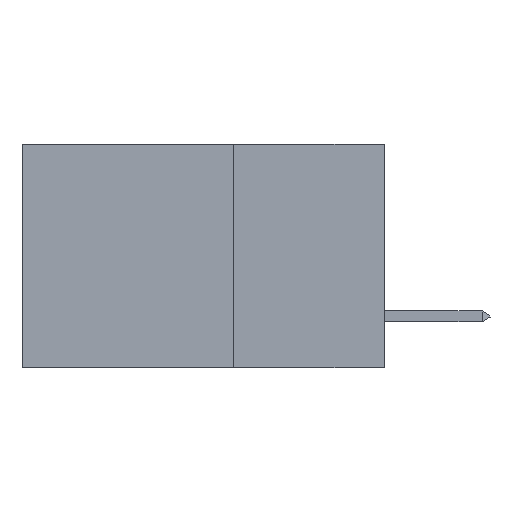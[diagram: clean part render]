
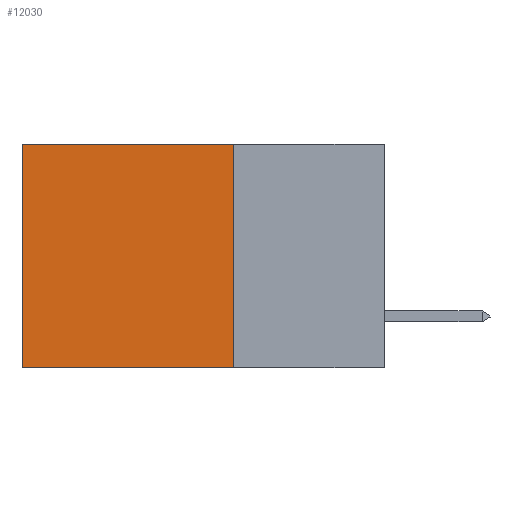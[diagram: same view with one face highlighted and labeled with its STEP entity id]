
A CAD part, left-side view. The second image highlights one B-rep face of the part: STEP entity #12030.
In plain terms, the highlighted planar face has unit normal (-1, 0, 0).
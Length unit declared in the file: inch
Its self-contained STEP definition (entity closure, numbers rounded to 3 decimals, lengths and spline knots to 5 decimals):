
#408 = CARTESIAN_POINT ( 'NONE',  ( 0.2875, 0.25, 0. ) ) ;
#1227 = FACE_OUTER_BOUND ( 'NONE', #35162, .T. ) ;
#2626 = LINE ( 'NONE', #7851, #26448 ) ;
#3284 = VERTEX_POINT ( 'NONE', #4721 ) ;
#3836 = DIRECTION ( 'NONE',  ( 0., 1., 0. ) ) ;
#4527 = PLANE ( 'NONE',  #27388 ) ;
#4721 = CARTESIAN_POINT ( 'NONE',  ( 0.2875, 0.25, -0.37 ) ) ;
#6178 = VECTOR ( 'NONE', #39153, 39.37008 ) ;
#7851 = CARTESIAN_POINT ( 'NONE',  ( 0.2875, 0.25, -0.37 ) ) ;
#7885 = VERTEX_POINT ( 'NONE', #36113 ) ;
#8228 = VECTOR ( 'NONE', #13707, 39.37008 ) ;
#8295 = EDGE_CURVE ( 'NONE', #7885, #3284, #20271, .T. ) ;
#10397 = DIRECTION ( 'NONE',  ( 0., 1., 0. ) ) ;
#12030 = ADVANCED_FACE ( 'NONE', ( #1227 ), #4527, .F. ) ;
#13108 = ORIENTED_EDGE ( 'NONE', *, *, #27573, .F. ) ;
#13623 = LINE ( 'NONE', #408, #18024 ) ;
#13707 = DIRECTION ( 'NONE',  ( 0., 0., -1. ) ) ;
#14038 = EDGE_CURVE ( 'NONE', #31736, #35917, #34046, .T. ) ;
#18024 = VECTOR ( 'NONE', #3836, 39.37008 ) ;
#19858 = ORIENTED_EDGE ( 'NONE', *, *, #8295, .F. ) ;
#20271 = LINE ( 'NONE', #28064, #6178 ) ;
#21760 = EDGE_CURVE ( 'NONE', #7885, #31736, #13623, .T. ) ;
#21918 = ORIENTED_EDGE ( 'NONE', *, *, #21760, .T. ) ;
#22974 = CARTESIAN_POINT ( 'NONE',  ( 0.2875, 0.6, 0. ) ) ;
#23714 = CARTESIAN_POINT ( 'NONE',  ( 0.2875, 0.25, 0. ) ) ;
#26448 = VECTOR ( 'NONE', #10397, 39.37008 ) ;
#27019 = ORIENTED_EDGE ( 'NONE', *, *, #14038, .T. ) ;
#27388 = AXIS2_PLACEMENT_3D ( 'NONE', #23714, #29791, #33226 ) ;
#27573 = EDGE_CURVE ( 'NONE', #3284, #35917, #2626, .T. ) ;
#28064 = CARTESIAN_POINT ( 'NONE',  ( 0.2875, 0.25, 0. ) ) ;
#29791 = DIRECTION ( 'NONE',  ( 1., 0., 0. ) ) ;
#31736 = VERTEX_POINT ( 'NONE', #33197 ) ;
#33197 = CARTESIAN_POINT ( 'NONE',  ( 0.2875, 0.6, 0. ) ) ;
#33226 = DIRECTION ( 'NONE',  ( 0., 0., -1. ) ) ;
#34046 = LINE ( 'NONE', #22974, #8228 ) ;
#35073 = CARTESIAN_POINT ( 'NONE',  ( 0.2875, 0.6, -0.37 ) ) ;
#35162 = EDGE_LOOP ( 'NONE', ( #27019, #13108, #19858, #21918 ) ) ;
#35917 = VERTEX_POINT ( 'NONE', #35073 ) ;
#36113 = CARTESIAN_POINT ( 'NONE',  ( 0.2875, 0.25, 0. ) ) ;
#39153 = DIRECTION ( 'NONE',  ( 0., 0., -1. ) ) ;
